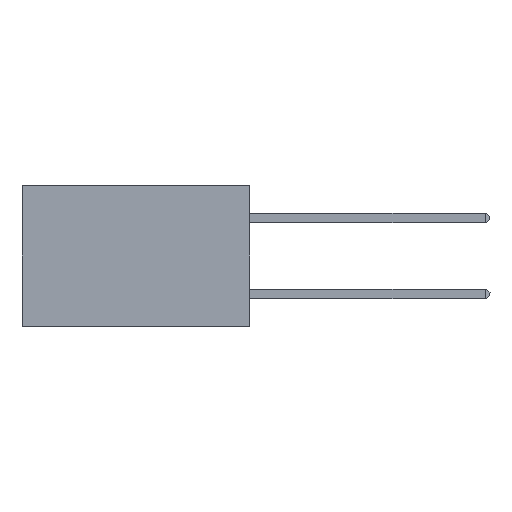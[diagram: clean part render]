
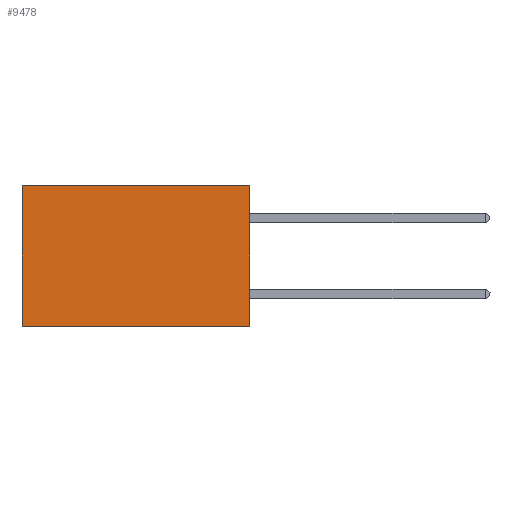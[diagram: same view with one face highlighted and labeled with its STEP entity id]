
A CAD part, left-side view. The second image highlights one B-rep face of the part: STEP entity #9478.
In plain terms, the highlighted planar face has unit normal (-1, 0, 0).
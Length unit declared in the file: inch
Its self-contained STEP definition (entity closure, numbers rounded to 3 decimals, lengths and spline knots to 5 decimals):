
#432 = EDGE_CURVE ( 'NONE', #3364, #6570, #7199, .T. ) ;
#572 = DIRECTION ( 'NONE',  ( 1., 0., 0. ) ) ;
#789 = EDGE_LOOP ( 'NONE', ( #3066, #5861, #3624, #1754 ) ) ;
#1435 = CARTESIAN_POINT ( 'NONE',  ( 0.2875, 0.6, 0. ) ) ;
#1754 = ORIENTED_EDGE ( 'NONE', *, *, #7941, .T. ) ;
#2022 = VERTEX_POINT ( 'NONE', #5190 ) ;
#2213 = DIRECTION ( 'NONE',  ( 0., 1., 0. ) ) ;
#2408 = CARTESIAN_POINT ( 'NONE',  ( 0.2875, 0.6, 0. ) ) ;
#2500 = CARTESIAN_POINT ( 'NONE',  ( 0.2875, 0., 0. ) ) ;
#2907 = DIRECTION ( 'NONE',  ( 0., 0., -1. ) ) ;
#2967 = EDGE_CURVE ( 'NONE', #5291, #6570, #5143, .T. ) ;
#3066 = ORIENTED_EDGE ( 'NONE', *, *, #432, .T. ) ;
#3252 = VECTOR ( 'NONE', #2213, 39.37008 ) ;
#3364 = VERTEX_POINT ( 'NONE', #1435 ) ;
#3450 = PLANE ( 'NONE',  #9077 ) ;
#3624 = ORIENTED_EDGE ( 'NONE', *, *, #4034, .F. ) ;
#4034 = EDGE_CURVE ( 'NONE', #2022, #5291, #9101, .T. ) ;
#4400 = CARTESIAN_POINT ( 'NONE',  ( 0.2875, 0., 0. ) ) ;
#4709 = FACE_OUTER_BOUND ( 'NONE', #789, .T. ) ;
#4786 = DIRECTION ( 'NONE',  ( 0., 1., 0. ) ) ;
#4969 = DIRECTION ( 'NONE',  ( 0., 0., -1. ) ) ;
#5143 = LINE ( 'NONE', #9737, #3252 ) ;
#5158 = VECTOR ( 'NONE', #6928, 39.37008 ) ;
#5190 = CARTESIAN_POINT ( 'NONE',  ( 0.2875, 0., 0. ) ) ;
#5291 = VERTEX_POINT ( 'NONE', #5388 ) ;
#5364 = VECTOR ( 'NONE', #4969, 39.37008 ) ;
#5388 = CARTESIAN_POINT ( 'NONE',  ( 0.2875, 0., -0.37 ) ) ;
#5861 = ORIENTED_EDGE ( 'NONE', *, *, #2967, .F. ) ;
#6470 = VECTOR ( 'NONE', #4786, 39.37008 ) ;
#6570 = VERTEX_POINT ( 'NONE', #9907 ) ;
#6928 = DIRECTION ( 'NONE',  ( 0., 0., -1. ) ) ;
#7199 = LINE ( 'NONE', #2408, #5158 ) ;
#7941 = EDGE_CURVE ( 'NONE', #2022, #3364, #9636, .T. ) ;
#8826 = CARTESIAN_POINT ( 'NONE',  ( 0.2875, 0., 0. ) ) ;
#9077 = AXIS2_PLACEMENT_3D ( 'NONE', #4400, #572, #2907 ) ;
#9101 = LINE ( 'NONE', #8826, #5364 ) ;
#9478 = ADVANCED_FACE ( 'NONE', ( #4709 ), #3450, .F. ) ;
#9636 = LINE ( 'NONE', #2500, #6470 ) ;
#9737 = CARTESIAN_POINT ( 'NONE',  ( 0.2875, 0., -0.37 ) ) ;
#9907 = CARTESIAN_POINT ( 'NONE',  ( 0.2875, 0.6, -0.37 ) ) ;
